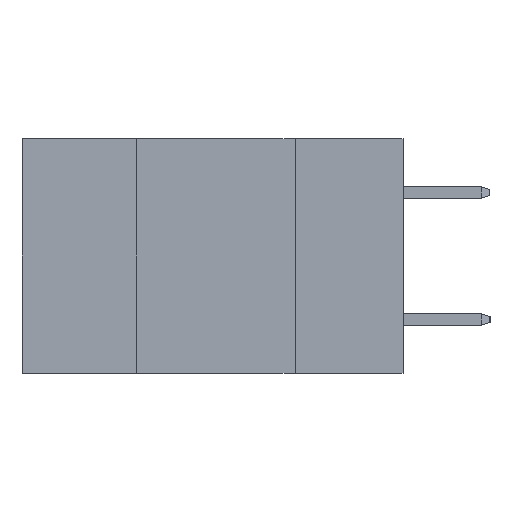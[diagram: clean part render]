
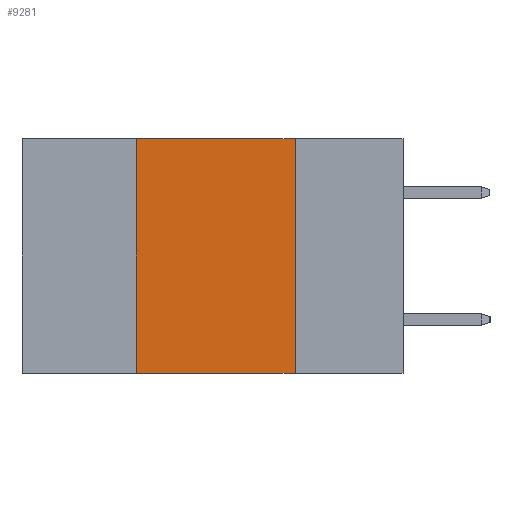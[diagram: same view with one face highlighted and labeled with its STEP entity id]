
A CAD part, left-side view. The second image highlights one B-rep face of the part: STEP entity #9281.
In plain terms, the highlighted planar face has unit normal (-1, 0, 0).
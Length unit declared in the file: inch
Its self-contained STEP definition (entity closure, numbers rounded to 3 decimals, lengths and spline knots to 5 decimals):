
#81 = CARTESIAN_POINT ( 'NONE',  ( 0., 0.6, -0.37 ) ) ;
#221 = LINE ( 'NONE', #9583, #9538 ) ;
#547 = VERTEX_POINT ( 'NONE', #10254 ) ;
#683 = DIRECTION ( 'NONE',  ( 1., 0., 0. ) ) ;
#1056 = DIRECTION ( 'NONE',  ( 0., -1., 0. ) ) ;
#1205 = VECTOR ( 'NONE', #3581, 39.37008 ) ;
#1431 = VECTOR ( 'NONE', #1056, 39.37008 ) ;
#1781 = AXIS2_PLACEMENT_3D ( 'NONE', #10903, #683, #9016 ) ;
#1917 = CARTESIAN_POINT ( 'NONE',  ( 0., 0.42, -0.37 ) ) ;
#2090 = ORIENTED_EDGE ( 'NONE', *, *, #9511, .F. ) ;
#2264 = ORIENTED_EDGE ( 'NONE', *, *, #4701, .T. ) ;
#3581 = DIRECTION ( 'NONE',  ( 0., 0., 1. ) ) ;
#3794 = LINE ( 'NONE', #7031, #10673 ) ;
#4243 = VERTEX_POINT ( 'NONE', #4413 ) ;
#4354 = CARTESIAN_POINT ( 'NONE',  ( 0., 0.42, 0. ) ) ;
#4408 = LINE ( 'NONE', #4354, #1205 ) ;
#4413 = CARTESIAN_POINT ( 'NONE',  ( 0., 0.17, -0.37 ) ) ;
#4701 = EDGE_CURVE ( 'NONE', #5631, #4243, #10276, .T. ) ;
#5244 = EDGE_CURVE ( 'NONE', #547, #4243, #221, .T. ) ;
#5333 = EDGE_LOOP ( 'NONE', ( #5339, #2090, #6921, #2264 ) ) ;
#5339 = ORIENTED_EDGE ( 'NONE', *, *, #5244, .F. ) ;
#5631 = VERTEX_POINT ( 'NONE', #1917 ) ;
#6654 = FACE_OUTER_BOUND ( 'NONE', #5333, .T. ) ;
#6921 = ORIENTED_EDGE ( 'NONE', *, *, #8993, .F. ) ;
#7031 = CARTESIAN_POINT ( 'NONE',  ( 0., 0.6, 0. ) ) ;
#7149 = DIRECTION ( 'NONE',  ( 0., -1., 0. ) ) ;
#7865 = DIRECTION ( 'NONE',  ( 0., 0., -1. ) ) ;
#7923 = VERTEX_POINT ( 'NONE', #10590 ) ;
#8993 = EDGE_CURVE ( 'NONE', #5631, #7923, #4408, .T. ) ;
#9016 = DIRECTION ( 'NONE',  ( 0., 0., -1. ) ) ;
#9281 = ADVANCED_FACE ( 'NONE', ( #6654 ), #10050, .F. ) ;
#9511 = EDGE_CURVE ( 'NONE', #7923, #547, #3794, .T. ) ;
#9538 = VECTOR ( 'NONE', #7865, 39.37008 ) ;
#9583 = CARTESIAN_POINT ( 'NONE',  ( 0., 0.17, 0. ) ) ;
#10050 = PLANE ( 'NONE',  #1781 ) ;
#10254 = CARTESIAN_POINT ( 'NONE',  ( 0., 0.17, 0. ) ) ;
#10276 = LINE ( 'NONE', #81, #1431 ) ;
#10590 = CARTESIAN_POINT ( 'NONE',  ( 0., 0.42, 0. ) ) ;
#10673 = VECTOR ( 'NONE', #7149, 39.37008 ) ;
#10903 = CARTESIAN_POINT ( 'NONE',  ( 0., 0.6, 0. ) ) ;
